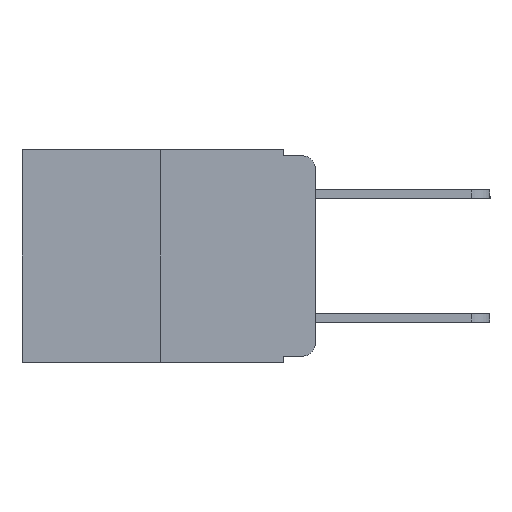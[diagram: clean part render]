
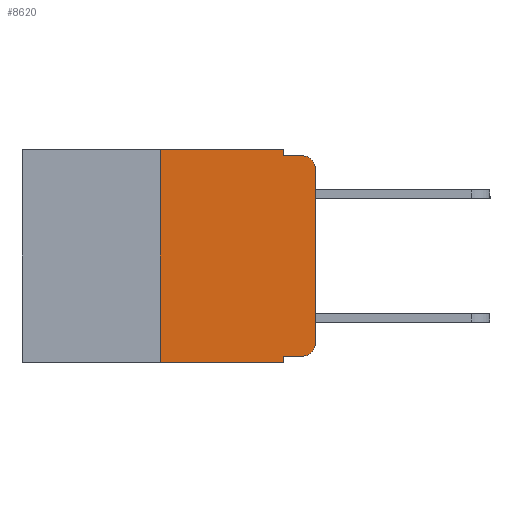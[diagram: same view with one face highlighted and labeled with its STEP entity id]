
A CAD part, left-side view. The second image highlights one B-rep face of the part: STEP entity #8620.
In plain terms, the highlighted planar face has unit normal (-1, 0, 0).
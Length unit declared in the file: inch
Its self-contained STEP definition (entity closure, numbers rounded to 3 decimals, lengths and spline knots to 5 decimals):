
#158 = EDGE_CURVE ( 'NONE', #2035, #8389, #5493, .T. ) ;
#180 = DIRECTION ( 'NONE',  ( -1., 0., 0. ) ) ;
#185 = ORIENTED_EDGE ( 'NONE', *, *, #5198, .F. ) ;
#202 = CARTESIAN_POINT ( 'NONE',  ( 0., 0.02, -0.313 ) ) ;
#583 = FACE_OUTER_BOUND ( 'NONE', #1817, .T. ) ;
#621 = CARTESIAN_POINT ( 'NONE',  ( 0., 0.25, 0. ) ) ;
#702 = CARTESIAN_POINT ( 'NONE',  ( 0., 0., -0.03 ) ) ;
#774 = VERTEX_POINT ( 'NONE', #9146 ) ;
#786 = DIRECTION ( 'NONE',  ( 0., 0., -1. ) ) ;
#893 = DIRECTION ( 'NONE',  ( 0., 0., -1. ) ) ;
#915 = ORIENTED_EDGE ( 'NONE', *, *, #7826, .F. ) ;
#1027 = EDGE_CURVE ( 'NONE', #4921, #7072, #5309, .T. ) ;
#1082 = VECTOR ( 'NONE', #6130, 39.37008 ) ;
#1817 = EDGE_LOOP ( 'NONE', ( #7789, #5478, #185, #5797, #915, #3838, #11780, #12297, #7625, #3033 ) ) ;
#1842 = CARTESIAN_POINT ( 'NONE',  ( 0., 0.051, -0.333 ) ) ;
#1958 = AXIS2_PLACEMENT_3D ( 'NONE', #202, #180, #893 ) ;
#2013 = DIRECTION ( 'NONE',  ( 0., 0., -1. ) ) ;
#2035 = VERTEX_POINT ( 'NONE', #4941 ) ;
#2625 = LINE ( 'NONE', #9322, #10154 ) ;
#2749 = DIRECTION ( 'NONE',  ( 0., -1., 0. ) ) ;
#2793 = VECTOR ( 'NONE', #2749, 39.37008 ) ;
#3007 = EDGE_CURVE ( 'NONE', #7334, #774, #4956, .T. ) ;
#3033 = ORIENTED_EDGE ( 'NONE', *, *, #3007, .T. ) ;
#3598 = CARTESIAN_POINT ( 'NONE',  ( 0., 0.051, -0.01 ) ) ;
#3645 = CARTESIAN_POINT ( 'NONE',  ( 0., 0.02, -0.333 ) ) ;
#3726 = VERTEX_POINT ( 'NONE', #5880 ) ;
#3838 = ORIENTED_EDGE ( 'NONE', *, *, #158, .F. ) ;
#3859 = VERTEX_POINT ( 'NONE', #3598 ) ;
#4551 = AXIS2_PLACEMENT_3D ( 'NONE', #9868, #9718, #9702 ) ;
#4610 = LINE ( 'NONE', #6498, #11978 ) ;
#4674 = CARTESIAN_POINT ( 'NONE',  ( 0., 0.473, -0.343 ) ) ;
#4721 = LINE ( 'NONE', #12419, #12082 ) ;
#4857 = VECTOR ( 'NONE', #12015, 39.37008 ) ;
#4921 = VERTEX_POINT ( 'NONE', #702 ) ;
#4941 = CARTESIAN_POINT ( 'NONE',  ( 0., 0.25, -0.343 ) ) ;
#4956 = CIRCLE ( 'NONE', #1958, 0.02 ) ;
#5001 = CARTESIAN_POINT ( 'NONE',  ( 0., 0.25, 0. ) ) ;
#5198 = EDGE_CURVE ( 'NONE', #3859, #7072, #2625, .T. ) ;
#5309 = CIRCLE ( 'NONE', #8056, 0.02 ) ;
#5478 = ORIENTED_EDGE ( 'NONE', *, *, #1027, .T. ) ;
#5493 = LINE ( 'NONE', #5001, #4857 ) ;
#5797 = ORIENTED_EDGE ( 'NONE', *, *, #10445, .F. ) ;
#5811 = EDGE_CURVE ( 'NONE', #6984, #8539, #4610, .T. ) ;
#5880 = CARTESIAN_POINT ( 'NONE',  ( 0., 0.051, 0. ) ) ;
#6130 = DIRECTION ( 'NONE',  ( 0., -1., 0. ) ) ;
#6477 = VECTOR ( 'NONE', #8554, 39.37008 ) ;
#6498 = CARTESIAN_POINT ( 'NONE',  ( 0., 0.051, 0. ) ) ;
#6848 = EDGE_CURVE ( 'NONE', #774, #4921, #4721, .T. ) ;
#6984 = VERTEX_POINT ( 'NONE', #1842 ) ;
#7072 = VERTEX_POINT ( 'NONE', #10561 ) ;
#7334 = VERTEX_POINT ( 'NONE', #3645 ) ;
#7625 = ORIENTED_EDGE ( 'NONE', *, *, #9809, .T. ) ;
#7789 = ORIENTED_EDGE ( 'NONE', *, *, #6848, .T. ) ;
#7826 = EDGE_CURVE ( 'NONE', #8389, #3726, #11568, .T. ) ;
#7930 = LINE ( 'NONE', #7956, #10760 ) ;
#7956 = CARTESIAN_POINT ( 'NONE',  ( 0., 0.051, 0. ) ) ;
#8056 = AXIS2_PLACEMENT_3D ( 'NONE', #9781, #10727, #10731 ) ;
#8389 = VERTEX_POINT ( 'NONE', #621 ) ;
#8539 = VERTEX_POINT ( 'NONE', #12803 ) ;
#8545 = DIRECTION ( 'NONE',  ( 0., 0., 1. ) ) ;
#8554 = DIRECTION ( 'NONE',  ( 0., -1., 0. ) ) ;
#8620 = ADVANCED_FACE ( 'NONE', ( #583 ), #9825, .F. ) ;
#9146 = CARTESIAN_POINT ( 'NONE',  ( 0., 0., -0.313 ) ) ;
#9166 = LINE ( 'NONE', #10947, #1082 ) ;
#9322 = CARTESIAN_POINT ( 'NONE',  ( 0., 0.051, -0.01 ) ) ;
#9702 = DIRECTION ( 'NONE',  ( 0., 0., -1. ) ) ;
#9718 = DIRECTION ( 'NONE',  ( 1., 0., 0. ) ) ;
#9781 = CARTESIAN_POINT ( 'NONE',  ( 0., 0.02, -0.03 ) ) ;
#9809 = EDGE_CURVE ( 'NONE', #6984, #7334, #9166, .T. ) ;
#9825 = PLANE ( 'NONE',  #4551 ) ;
#9868 = CARTESIAN_POINT ( 'NONE',  ( 0., 0.473, 0. ) ) ;
#10154 = VECTOR ( 'NONE', #10447, 39.37008 ) ;
#10445 = EDGE_CURVE ( 'NONE', #3726, #3859, #7930, .T. ) ;
#10447 = DIRECTION ( 'NONE',  ( 0., -1., 0. ) ) ;
#10561 = CARTESIAN_POINT ( 'NONE',  ( 0., 0.02, -0.01 ) ) ;
#10592 = LINE ( 'NONE', #4674, #2793 ) ;
#10727 = DIRECTION ( 'NONE',  ( -1., 0., 0. ) ) ;
#10731 = DIRECTION ( 'NONE',  ( 0., 0., -1. ) ) ;
#10760 = VECTOR ( 'NONE', #786, 39.37008 ) ;
#10851 = CARTESIAN_POINT ( 'NONE',  ( 0., 0.473, 0. ) ) ;
#10947 = CARTESIAN_POINT ( 'NONE',  ( 0., 0.051, -0.333 ) ) ;
#11428 = EDGE_CURVE ( 'NONE', #2035, #8539, #10592, .T. ) ;
#11568 = LINE ( 'NONE', #10851, #6477 ) ;
#11780 = ORIENTED_EDGE ( 'NONE', *, *, #11428, .T. ) ;
#11978 = VECTOR ( 'NONE', #2013, 39.37008 ) ;
#12015 = DIRECTION ( 'NONE',  ( 0., 0., 1. ) ) ;
#12082 = VECTOR ( 'NONE', #8545, 39.37008 ) ;
#12297 = ORIENTED_EDGE ( 'NONE', *, *, #5811, .F. ) ;
#12419 = CARTESIAN_POINT ( 'NONE',  ( 0., 0., 0. ) ) ;
#12803 = CARTESIAN_POINT ( 'NONE',  ( 0., 0.051, -0.343 ) ) ;
